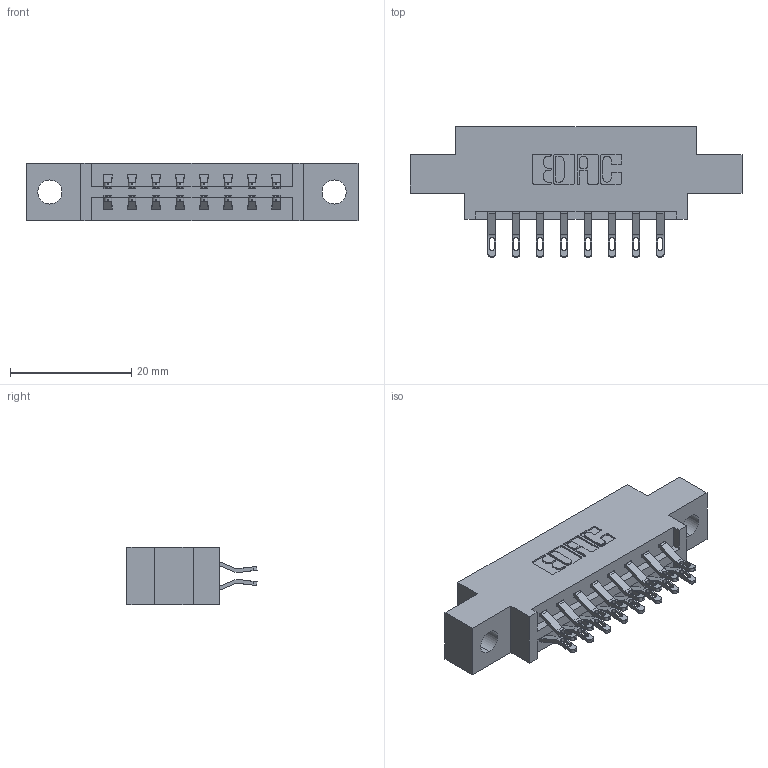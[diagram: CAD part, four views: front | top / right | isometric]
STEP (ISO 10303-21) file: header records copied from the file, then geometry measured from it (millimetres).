
FILE_DESCRIPTION (( 'STEP AP203' ), '1' );
FILE_NAME ('337-016-555-804.STEP', '2019-10-10T18:14:10', ( '' ), ( '' ), 'SwSTEP 2.0', 'SolidWorks 2016', '' );
FILE_SCHEMA (( 'CONFIG_CONTROL_DESIGN' ));
Length unit declared in the file: inch
Products named in the file (3): 345-292-001_555 Tail; 337 Part_0.170 Offset - 0.156 Dia-TH; 337-016-555-804
Assembly tree (17 placements, depth 2):
  337-016-555-804
    337 Part_0.170 Offset - 0.156 Dia-TH
    345-292-001_555 Tail  x16
Bounding box: 54.71 x 21.47 x 9.4 mm (x, y, z)
Volume: 5154.4 mm3; surface area: 5576.9 mm2
Topology: 17 solids, 17 shells, 1078 faces, 3347 edges, 2230 vertices
Faces by surface type: plane 650, cylinder 428
Entity records: 11061 total; most frequent: CARTESIAN_POINT 1928, ORIENTED_EDGE 1834, DIRECTION 1673, EDGE_CURVE 917, LINE 769, VECTOR 769, VERTEX_POINT 610, AXIS2_PLACEMENT_3D 452
